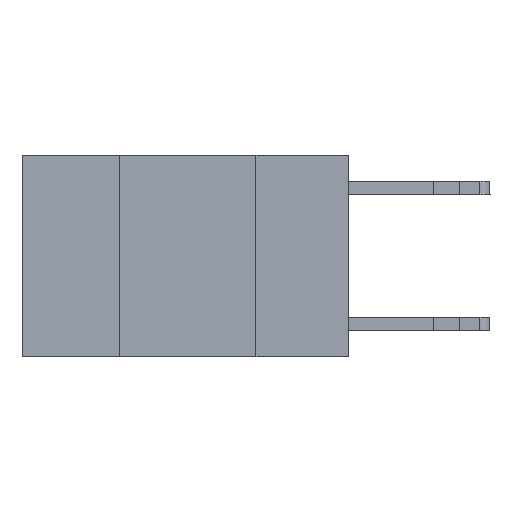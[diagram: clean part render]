
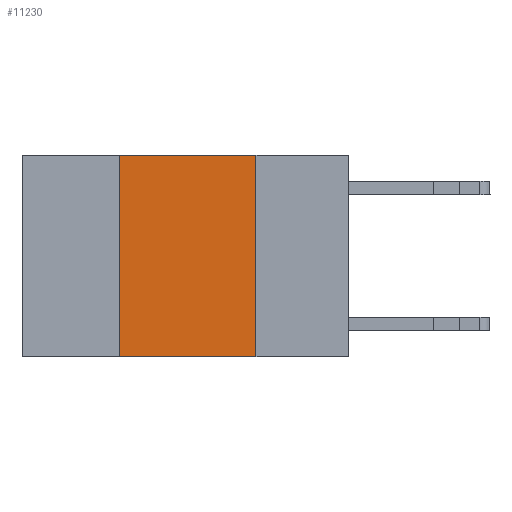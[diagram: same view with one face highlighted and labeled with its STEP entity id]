
A CAD part, left-side view. The second image highlights one B-rep face of the part: STEP entity #11230.
In plain terms, the highlighted planar face has unit normal (-1, 0, 0).
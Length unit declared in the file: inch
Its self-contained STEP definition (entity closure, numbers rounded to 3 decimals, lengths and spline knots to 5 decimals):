
#209 = EDGE_CURVE ( 'NONE', #5905, #9248, #7415, .T. ) ;
#358 = EDGE_CURVE ( 'NONE', #4545, #19397, #5367, .T. ) ;
#1177 = EDGE_CURVE ( 'NONE', #4545, #9248, #13022, .T. ) ;
#3558 = PLANE ( 'NONE',  #9749 ) ;
#4545 = VERTEX_POINT ( 'NONE', #7504 ) ;
#4798 = DIRECTION ( 'NONE',  ( 0., 0., -1. ) ) ;
#4887 = DIRECTION ( 'NONE',  ( 1., 0., 0. ) ) ;
#5007 = FACE_OUTER_BOUND ( 'NONE', #13655, .T. ) ;
#5052 = VECTOR ( 'NONE', #14283, 39.37008 ) ;
#5367 = LINE ( 'NONE', #17866, #5052 ) ;
#5905 = VERTEX_POINT ( 'NONE', #14674 ) ;
#6301 = CARTESIAN_POINT ( 'NONE',  ( 0., 0.17, 0. ) ) ;
#6952 = CARTESIAN_POINT ( 'NONE',  ( 0., 0.17, -0.37 ) ) ;
#7263 = VECTOR ( 'NONE', #11748, 39.37008 ) ;
#7415 = LINE ( 'NONE', #6301, #7263 ) ;
#7504 = CARTESIAN_POINT ( 'NONE',  ( 0., 0.42, -0.37 ) ) ;
#8482 = CARTESIAN_POINT ( 'NONE',  ( 0., 0.6, 0. ) ) ;
#9153 = ORIENTED_EDGE ( 'NONE', *, *, #209, .F. ) ;
#9248 = VERTEX_POINT ( 'NONE', #6952 ) ;
#9393 = ORIENTED_EDGE ( 'NONE', *, *, #20141, .F. ) ;
#9508 = ORIENTED_EDGE ( 'NONE', *, *, #358, .F. ) ;
#9749 = AXIS2_PLACEMENT_3D ( 'NONE', #8482, #4887, #4798 ) ;
#9800 = CARTESIAN_POINT ( 'NONE',  ( 0., 0.42, 0. ) ) ;
#9932 = ORIENTED_EDGE ( 'NONE', *, *, #1177, .T. ) ;
#10626 = VECTOR ( 'NONE', #17209, 39.37008 ) ;
#10654 = LINE ( 'NONE', #17150, #10626 ) ;
#11230 = ADVANCED_FACE ( 'NONE', ( #5007 ), #3558, .F. ) ;
#11748 = DIRECTION ( 'NONE',  ( 0., 0., -1. ) ) ;
#12036 = CARTESIAN_POINT ( 'NONE',  ( 0., 0.6, -0.37 ) ) ;
#12703 = DIRECTION ( 'NONE',  ( 0., -1., 0. ) ) ;
#13022 = LINE ( 'NONE', #12036, #13307 ) ;
#13307 = VECTOR ( 'NONE', #12703, 39.37008 ) ;
#13655 = EDGE_LOOP ( 'NONE', ( #9153, #9393, #9508, #9932 ) ) ;
#14283 = DIRECTION ( 'NONE',  ( 0., 0., 1. ) ) ;
#14674 = CARTESIAN_POINT ( 'NONE',  ( 0., 0.17, 0. ) ) ;
#17150 = CARTESIAN_POINT ( 'NONE',  ( 0., 0.6, 0. ) ) ;
#17209 = DIRECTION ( 'NONE',  ( 0., -1., 0. ) ) ;
#17866 = CARTESIAN_POINT ( 'NONE',  ( 0., 0.42, 0. ) ) ;
#19397 = VERTEX_POINT ( 'NONE', #9800 ) ;
#20141 = EDGE_CURVE ( 'NONE', #19397, #5905, #10654, .T. ) ;
